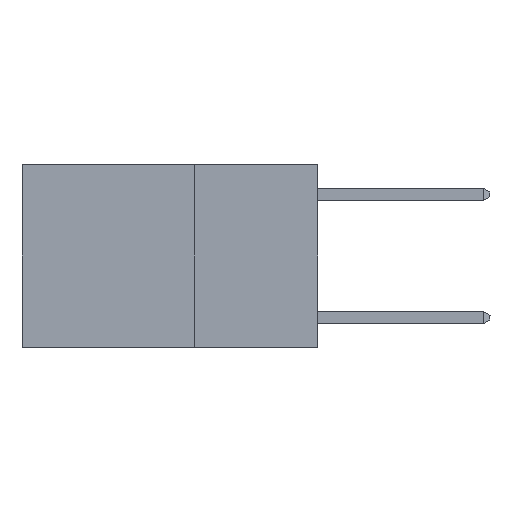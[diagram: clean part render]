
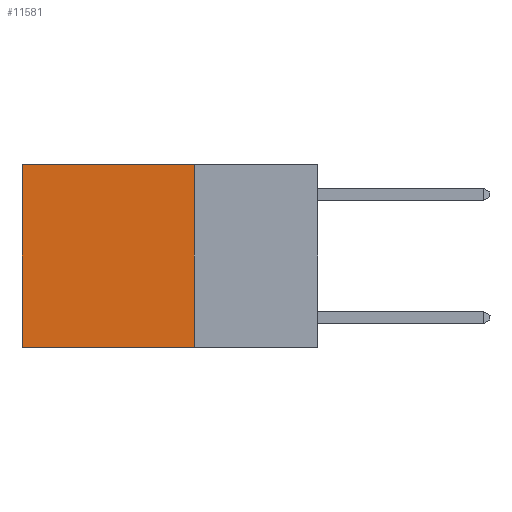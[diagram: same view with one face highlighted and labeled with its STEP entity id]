
A CAD part, left-side view. The second image highlights one B-rep face of the part: STEP entity #11581.
In plain terms, the highlighted planar face has unit normal (-1, 0, 0).
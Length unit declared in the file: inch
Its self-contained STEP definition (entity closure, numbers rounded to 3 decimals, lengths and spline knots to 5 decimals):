
#499 = VECTOR ( 'NONE', #18561, 39.37008 ) ;
#901 = PLANE ( 'NONE',  #3554 ) ;
#2008 = CARTESIAN_POINT ( 'NONE',  ( 0.2625, 0.25, 0. ) ) ;
#2687 = DIRECTION ( 'NONE',  ( 0., 0., -1. ) ) ;
#3136 = VECTOR ( 'NONE', #21602, 39.37008 ) ;
#3554 = AXIS2_PLACEMENT_3D ( 'NONE', #21626, #13074, #2687 ) ;
#3865 = VERTEX_POINT ( 'NONE', #7981 ) ;
#5235 = VECTOR ( 'NONE', #8921, 39.37008 ) ;
#5870 = CARTESIAN_POINT ( 'NONE',  ( 0.2625, 0.6, 0. ) ) ;
#6141 = ORIENTED_EDGE ( 'NONE', *, *, #15871, .F. ) ;
#6586 = VERTEX_POINT ( 'NONE', #21285 ) ;
#7197 = CARTESIAN_POINT ( 'NONE',  ( 0.2625, 0.6, 0. ) ) ;
#7981 = CARTESIAN_POINT ( 'NONE',  ( 0.2625, 0.25, 0. ) ) ;
#8134 = CARTESIAN_POINT ( 'NONE',  ( 0.2625, 0.6, -0.37 ) ) ;
#8802 = EDGE_CURVE ( 'NONE', #3865, #16380, #16639, .T. ) ;
#8921 = DIRECTION ( 'NONE',  ( 0., 0., -1. ) ) ;
#9529 = ORIENTED_EDGE ( 'NONE', *, *, #8802, .T. ) ;
#9578 = CARTESIAN_POINT ( 'NONE',  ( 0.2625, 0.25, 0. ) ) ;
#9861 = LINE ( 'NONE', #7197, #5235 ) ;
#11581 = ADVANCED_FACE ( 'NONE', ( #20740 ), #901, .F. ) ;
#11809 = LINE ( 'NONE', #9578, #3136 ) ;
#12293 = EDGE_CURVE ( 'NONE', #3865, #6586, #11809, .T. ) ;
#13074 = DIRECTION ( 'NONE',  ( 1., 0., 0. ) ) ;
#14397 = ORIENTED_EDGE ( 'NONE', *, *, #20709, .T. ) ;
#14422 = LINE ( 'NONE', #16831, #499 ) ;
#14459 = EDGE_LOOP ( 'NONE', ( #14397, #6141, #21952, #9529 ) ) ;
#15537 = VECTOR ( 'NONE', #19369, 39.37008 ) ;
#15871 = EDGE_CURVE ( 'NONE', #6586, #21741, #14422, .T. ) ;
#16380 = VERTEX_POINT ( 'NONE', #5870 ) ;
#16639 = LINE ( 'NONE', #2008, #15537 ) ;
#16831 = CARTESIAN_POINT ( 'NONE',  ( 0.2625, 0.25, -0.37 ) ) ;
#18561 = DIRECTION ( 'NONE',  ( 0., 1., 0. ) ) ;
#19369 = DIRECTION ( 'NONE',  ( 0., 1., 0. ) ) ;
#20709 = EDGE_CURVE ( 'NONE', #16380, #21741, #9861, .T. ) ;
#20740 = FACE_OUTER_BOUND ( 'NONE', #14459, .T. ) ;
#21285 = CARTESIAN_POINT ( 'NONE',  ( 0.2625, 0.25, -0.37 ) ) ;
#21602 = DIRECTION ( 'NONE',  ( 0., 0., -1. ) ) ;
#21626 = CARTESIAN_POINT ( 'NONE',  ( 0.2625, 0.25, 0. ) ) ;
#21741 = VERTEX_POINT ( 'NONE', #8134 ) ;
#21952 = ORIENTED_EDGE ( 'NONE', *, *, #12293, .F. ) ;
